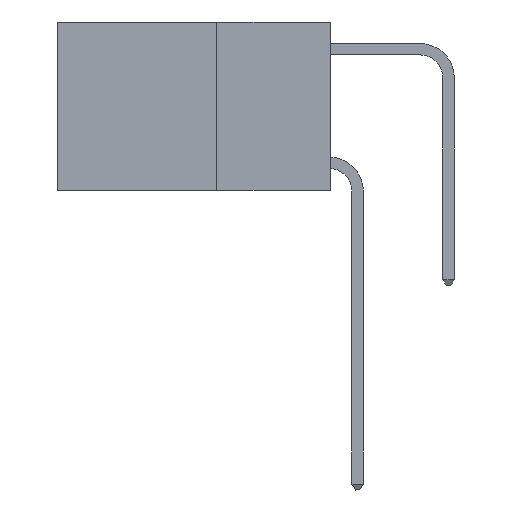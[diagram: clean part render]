
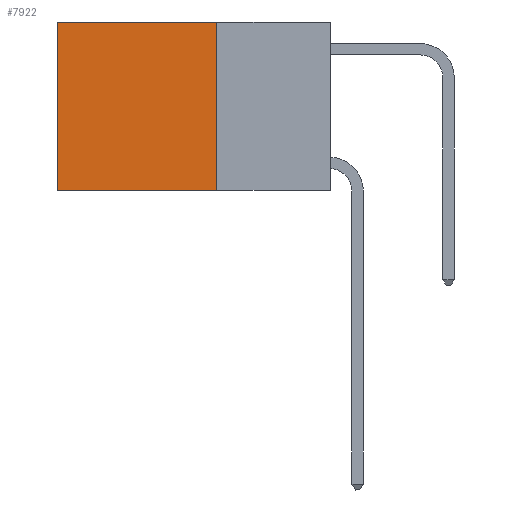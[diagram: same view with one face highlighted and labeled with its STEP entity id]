
A CAD part, left-side view. The second image highlights one B-rep face of the part: STEP entity #7922.
In plain terms, the highlighted planar face has unit normal (-1, 0, 0).
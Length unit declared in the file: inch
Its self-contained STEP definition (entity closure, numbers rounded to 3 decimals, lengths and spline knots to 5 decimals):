
#350 = LINE ( 'NONE', #7515, #7192 ) ;
#359 = CARTESIAN_POINT ( 'NONE',  ( 0.2625, 0.6, 0. ) ) ;
#361 = EDGE_CURVE ( 'NONE', #5274, #2844, #10124, .T. ) ;
#786 = DIRECTION ( 'NONE',  ( 0., 0., -1. ) ) ;
#1539 = LINE ( 'NONE', #7582, #7733 ) ;
#1551 = DIRECTION ( 'NONE',  ( 1., 0., 0. ) ) ;
#1817 = CARTESIAN_POINT ( 'NONE',  ( 0.2625, 0.25, 0. ) ) ;
#1915 = ORIENTED_EDGE ( 'NONE', *, *, #7413, .T. ) ;
#2095 = VERTEX_POINT ( 'NONE', #359 ) ;
#2844 = VERTEX_POINT ( 'NONE', #9334 ) ;
#2999 = DIRECTION ( 'NONE',  ( 0., 1., 0. ) ) ;
#3360 = DIRECTION ( 'NONE',  ( 0., 1., 0. ) ) ;
#3601 = VECTOR ( 'NONE', #2999, 39.37008 ) ;
#3692 = EDGE_LOOP ( 'NONE', ( #1915, #9648, #6087, #8038 ) ) ;
#4665 = DIRECTION ( 'NONE',  ( 0., 0., -1. ) ) ;
#5045 = PLANE ( 'NONE',  #9764 ) ;
#5274 = VERTEX_POINT ( 'NONE', #7114 ) ;
#6087 = ORIENTED_EDGE ( 'NONE', *, *, #10625, .F. ) ;
#6888 = CARTESIAN_POINT ( 'NONE',  ( 0.2625, 0.25, -0.37 ) ) ;
#7040 = VECTOR ( 'NONE', #4665, 39.37008 ) ;
#7114 = CARTESIAN_POINT ( 'NONE',  ( 0.2625, 0.25, -0.37 ) ) ;
#7192 = VECTOR ( 'NONE', #3360, 39.37008 ) ;
#7413 = EDGE_CURVE ( 'NONE', #2095, #2844, #1539, .T. ) ;
#7430 = CARTESIAN_POINT ( 'NONE',  ( 0.2625, 0.25, 0. ) ) ;
#7466 = DIRECTION ( 'NONE',  ( 0., 0., -1. ) ) ;
#7515 = CARTESIAN_POINT ( 'NONE',  ( 0.2625, 0.25, 0. ) ) ;
#7582 = CARTESIAN_POINT ( 'NONE',  ( 0.2625, 0.6, 0. ) ) ;
#7733 = VECTOR ( 'NONE', #786, 39.37008 ) ;
#7922 = ADVANCED_FACE ( 'NONE', ( #10786 ), #5045, .F. ) ;
#8038 = ORIENTED_EDGE ( 'NONE', *, *, #9326, .T. ) ;
#8956 = LINE ( 'NONE', #9537, #7040 ) ;
#9326 = EDGE_CURVE ( 'NONE', #9459, #2095, #350, .T. ) ;
#9334 = CARTESIAN_POINT ( 'NONE',  ( 0.2625, 0.6, -0.37 ) ) ;
#9459 = VERTEX_POINT ( 'NONE', #1817 ) ;
#9537 = CARTESIAN_POINT ( 'NONE',  ( 0.2625, 0.25, 0. ) ) ;
#9648 = ORIENTED_EDGE ( 'NONE', *, *, #361, .F. ) ;
#9764 = AXIS2_PLACEMENT_3D ( 'NONE', #7430, #1551, #7466 ) ;
#10124 = LINE ( 'NONE', #6888, #3601 ) ;
#10625 = EDGE_CURVE ( 'NONE', #9459, #5274, #8956, .T. ) ;
#10786 = FACE_OUTER_BOUND ( 'NONE', #3692, .T. ) ;
